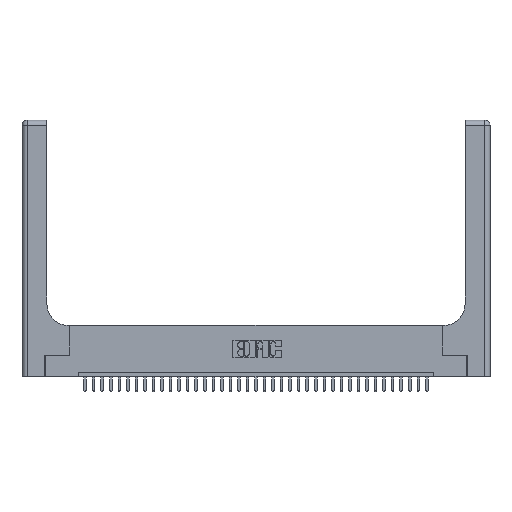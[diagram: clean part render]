
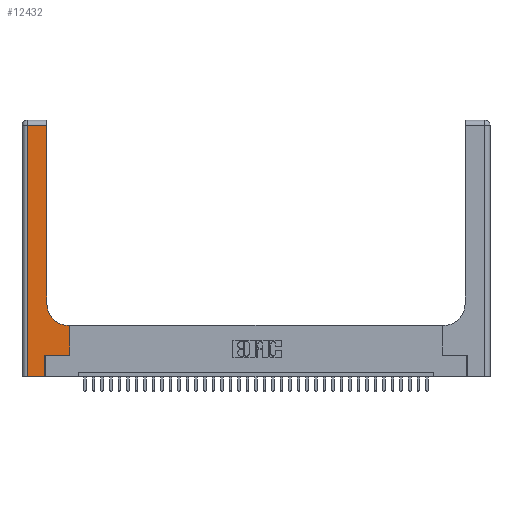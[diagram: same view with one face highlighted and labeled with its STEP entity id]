
A CAD part, top view. The second image highlights one B-rep face of the part: STEP entity #12432.
In plain terms, the highlighted planar face has unit normal (0, 0, 1).
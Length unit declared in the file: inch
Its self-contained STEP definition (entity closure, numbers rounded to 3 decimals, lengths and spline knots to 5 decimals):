
#127 = ORIENTED_EDGE ( 'NONE', *, *, #33847, .T. ) ;
#303 = VERTEX_POINT ( 'NONE', #8990 ) ;
#770 = DIRECTION ( 'NONE',  ( 0., 1., 0. ) ) ;
#1078 = LINE ( 'NONE', #11458, #25104 ) ;
#1175 = VERTEX_POINT ( 'NONE', #12470 ) ;
#1427 = ORIENTED_EDGE ( 'NONE', *, *, #18437, .T. ) ;
#1436 = VECTOR ( 'NONE', #30502, 39.37008 ) ;
#1903 = ORIENTED_EDGE ( 'NONE', *, *, #17314, .T. ) ;
#2922 = DIRECTION ( 'NONE',  ( 0., 1., 0. ) ) ;
#3409 = VERTEX_POINT ( 'NONE', #32354 ) ;
#4318 = EDGE_LOOP ( 'NONE', ( #28059, #17649, #16778, #1903, #1427, #21164, #13410, #16406, #127 ) ) ;
#4524 = EDGE_CURVE ( 'NONE', #4534, #26499, #26108, .T. ) ;
#4534 = VERTEX_POINT ( 'NONE', #28793 ) ;
#5256 = VERTEX_POINT ( 'NONE', #25165 ) ;
#5763 = CARTESIAN_POINT ( 'NONE',  ( 0., 3., 0.37 ) ) ;
#7203 = VERTEX_POINT ( 'NONE', #12550 ) ;
#8347 = CARTESIAN_POINT ( 'NONE',  ( 0.2915, 0.6, 0.37 ) ) ;
#8990 = CARTESIAN_POINT ( 'NONE',  ( 0.5415, 0.6, 0.37 ) ) ;
#10583 = EDGE_CURVE ( 'NONE', #26499, #32052, #27233, .T. ) ;
#10720 = VECTOR ( 'NONE', #2922, 39.37008 ) ;
#11458 = CARTESIAN_POINT ( 'NONE',  ( 0.2915, 3., 0.37 ) ) ;
#11965 = DIRECTION ( 'NONE',  ( 0., 0., -1. ) ) ;
#12285 = CARTESIAN_POINT ( 'NONE',  ( 0.269, 0., 0.37 ) ) ;
#12432 = ADVANCED_FACE ( 'NONE', ( #21897 ), #22074, .F. ) ;
#12470 = CARTESIAN_POINT ( 'NONE',  ( 0.5585, 0.6, 0.37 ) ) ;
#12550 = CARTESIAN_POINT ( 'NONE',  ( 0.269, 0., 0.37 ) ) ;
#13410 = ORIENTED_EDGE ( 'NONE', *, *, #26892, .T. ) ;
#13632 = LINE ( 'NONE', #32865, #24115 ) ;
#14201 = LINE ( 'NONE', #30596, #10720 ) ;
#14401 = LINE ( 'NONE', #12285, #32405 ) ;
#15034 = VECTOR ( 'NONE', #22158, 39.37008 ) ;
#15760 = VECTOR ( 'NONE', #29185, 39.37008 ) ;
#16406 = ORIENTED_EDGE ( 'NONE', *, *, #28140, .T. ) ;
#16596 = DIRECTION ( 'NONE',  ( 0., 0., -1. ) ) ;
#16778 = ORIENTED_EDGE ( 'NONE', *, *, #10583, .T. ) ;
#17314 = EDGE_CURVE ( 'NONE', #32052, #7203, #13632, .T. ) ;
#17325 = CARTESIAN_POINT ( 'NONE',  ( 0.269, 0.25, 0.37 ) ) ;
#17649 = ORIENTED_EDGE ( 'NONE', *, *, #4524, .T. ) ;
#18437 = EDGE_CURVE ( 'NONE', #7203, #18654, #14401, .T. ) ;
#18654 = VERTEX_POINT ( 'NONE', #17325 ) ;
#19365 = DIRECTION ( 'NONE',  ( -1., 0., 0. ) ) ;
#20389 = CARTESIAN_POINT ( 'NONE',  ( 0.5415, 0.85, 0.37 ) ) ;
#21164 = ORIENTED_EDGE ( 'NONE', *, *, #35910, .T. ) ;
#21897 = FACE_OUTER_BOUND ( 'NONE', #4318, .T. ) ;
#22074 = PLANE ( 'NONE',  #22654 ) ;
#22158 = DIRECTION ( 'NONE',  ( 0., -1., 0. ) ) ;
#22280 = CARTESIAN_POINT ( 'NONE',  ( 0.06, 3., 0.37 ) ) ;
#22654 = AXIS2_PLACEMENT_3D ( 'NONE', #5763, #16596, #19365 ) ;
#23077 = DIRECTION ( 'NONE',  ( 1., 0., 0. ) ) ;
#24115 = VECTOR ( 'NONE', #32981, 39.37008 ) ;
#25104 = VECTOR ( 'NONE', #33638, 39.37008 ) ;
#25165 = CARTESIAN_POINT ( 'NONE',  ( 0.5585, 0.25, 0.37 ) ) ;
#25891 = CARTESIAN_POINT ( 'NONE',  ( 0.06, 2.94, 0.37 ) ) ;
#25965 = DIRECTION ( 'NONE',  ( -1., 0., 0. ) ) ;
#26108 = LINE ( 'NONE', #34622, #34514 ) ;
#26499 = VERTEX_POINT ( 'NONE', #25891 ) ;
#26892 = EDGE_CURVE ( 'NONE', #5256, #1175, #14201, .T. ) ;
#27233 = LINE ( 'NONE', #22280, #15034 ) ;
#27651 = LINE ( 'NONE', #8347, #1436 ) ;
#28059 = ORIENTED_EDGE ( 'NONE', *, *, #29692, .T. ) ;
#28140 = EDGE_CURVE ( 'NONE', #1175, #303, #27651, .T. ) ;
#28793 = CARTESIAN_POINT ( 'NONE',  ( 0.2915, 2.94, 0.37 ) ) ;
#29185 = DIRECTION ( 'NONE',  ( 1., 0., 0. ) ) ;
#29401 = CIRCLE ( 'NONE', #29925, 0.25 ) ;
#29692 = EDGE_CURVE ( 'NONE', #3409, #4534, #1078, .T. ) ;
#29925 = AXIS2_PLACEMENT_3D ( 'NONE', #20389, #11965, #23077 ) ;
#30502 = DIRECTION ( 'NONE',  ( -1., 0., 0. ) ) ;
#30596 = CARTESIAN_POINT ( 'NONE',  ( 0.5585, 0.25, 0.37 ) ) ;
#31402 = CARTESIAN_POINT ( 'NONE',  ( 0.06, 0., 0.37 ) ) ;
#31497 = LINE ( 'NONE', #32281, #15760 ) ;
#32052 = VERTEX_POINT ( 'NONE', #31402 ) ;
#32281 = CARTESIAN_POINT ( 'NONE',  ( 0.269, 0.25, 0.37 ) ) ;
#32354 = CARTESIAN_POINT ( 'NONE',  ( 0.2915, 0.85, 0.37 ) ) ;
#32405 = VECTOR ( 'NONE', #770, 39.37008 ) ;
#32865 = CARTESIAN_POINT ( 'NONE',  ( 0., 0., 0.37 ) ) ;
#32981 = DIRECTION ( 'NONE',  ( 1., 0., 0. ) ) ;
#33638 = DIRECTION ( 'NONE',  ( 0., 1., 0. ) ) ;
#33847 = EDGE_CURVE ( 'NONE', #303, #3409, #29401, .T. ) ;
#34514 = VECTOR ( 'NONE', #25965, 39.37008 ) ;
#34622 = CARTESIAN_POINT ( 'NONE',  ( 0., 2.94, 0.37 ) ) ;
#35910 = EDGE_CURVE ( 'NONE', #18654, #5256, #31497, .T. ) ;
